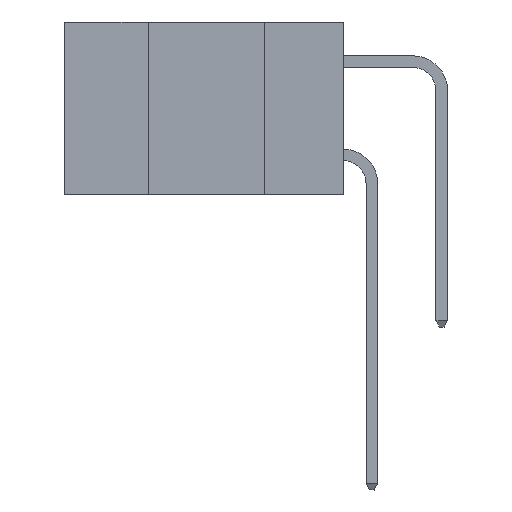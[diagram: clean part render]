
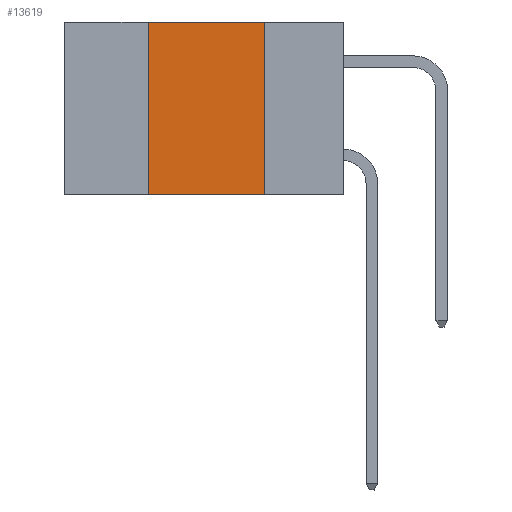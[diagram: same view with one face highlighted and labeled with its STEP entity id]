
A CAD part, left-side view. The second image highlights one B-rep face of the part: STEP entity #13619.
In plain terms, the highlighted planar face has unit normal (-1, 0, 0).
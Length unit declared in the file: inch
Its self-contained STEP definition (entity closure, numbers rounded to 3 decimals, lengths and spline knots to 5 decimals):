
#586 = VECTOR ( 'NONE', #5233, 39.37008 ) ;
#991 = CARTESIAN_POINT ( 'NONE',  ( 0., 0.6, 0. ) ) ;
#1155 = LINE ( 'NONE', #2580, #586 ) ;
#1272 = DIRECTION ( 'NONE',  ( 1., 0., 0. ) ) ;
#1414 = LINE ( 'NONE', #1505, #15227 ) ;
#1505 = CARTESIAN_POINT ( 'NONE',  ( 0., 0.17, -0.37 ) ) ;
#2580 = CARTESIAN_POINT ( 'NONE',  ( 0., 0.42, -0.37 ) ) ;
#2724 = VECTOR ( 'NONE', #9334, 39.37008 ) ;
#2995 = ORIENTED_EDGE ( 'NONE', *, *, #6769, .F. ) ;
#5039 = CARTESIAN_POINT ( 'NONE',  ( 0., 0.17, -0.37 ) ) ;
#5233 = DIRECTION ( 'NONE',  ( 0., 0., 1. ) ) ;
#5379 = CARTESIAN_POINT ( 'NONE',  ( 0., 0.42, 0. ) ) ;
#5697 = VERTEX_POINT ( 'NONE', #5379 ) ;
#6769 = EDGE_CURVE ( 'NONE', #11907, #5697, #1155, .T. ) ;
#7039 = DIRECTION ( 'NONE',  ( 0., 0., -1. ) ) ;
#8254 = ORIENTED_EDGE ( 'NONE', *, *, #17183, .F. ) ;
#8714 = EDGE_CURVE ( 'NONE', #11907, #18157, #16155, .T. ) ;
#8930 = ORIENTED_EDGE ( 'NONE', *, *, #8714, .T. ) ;
#9046 = CARTESIAN_POINT ( 'NONE',  ( 0., 0.6, -0.37 ) ) ;
#9334 = DIRECTION ( 'NONE',  ( 0., -1., 0. ) ) ;
#9422 = VECTOR ( 'NONE', #15275, 39.37008 ) ;
#10230 = EDGE_LOOP ( 'NONE', ( #18441, #8254, #2995, #8930 ) ) ;
#11452 = EDGE_CURVE ( 'NONE', #16791, #18157, #1414, .T. ) ;
#11907 = VERTEX_POINT ( 'NONE', #14604 ) ;
#12154 = LINE ( 'NONE', #15172, #9422 ) ;
#12259 = AXIS2_PLACEMENT_3D ( 'NONE', #991, #1272, #7039 ) ;
#12431 = FACE_OUTER_BOUND ( 'NONE', #10230, .T. ) ;
#13301 = DIRECTION ( 'NONE',  ( 0., 0., -1. ) ) ;
#13619 = ADVANCED_FACE ( 'NONE', ( #12431 ), #16793, .F. ) ;
#13972 = CARTESIAN_POINT ( 'NONE',  ( 0., 0.17, 0. ) ) ;
#14604 = CARTESIAN_POINT ( 'NONE',  ( 0., 0.42, -0.37 ) ) ;
#15172 = CARTESIAN_POINT ( 'NONE',  ( 0., 0.6, 0. ) ) ;
#15227 = VECTOR ( 'NONE', #13301, 39.37008 ) ;
#15275 = DIRECTION ( 'NONE',  ( 0., -1., 0. ) ) ;
#16155 = LINE ( 'NONE', #9046, #2724 ) ;
#16791 = VERTEX_POINT ( 'NONE', #13972 ) ;
#16793 = PLANE ( 'NONE',  #12259 ) ;
#17183 = EDGE_CURVE ( 'NONE', #5697, #16791, #12154, .T. ) ;
#18157 = VERTEX_POINT ( 'NONE', #5039 ) ;
#18441 = ORIENTED_EDGE ( 'NONE', *, *, #11452, .F. ) ;
